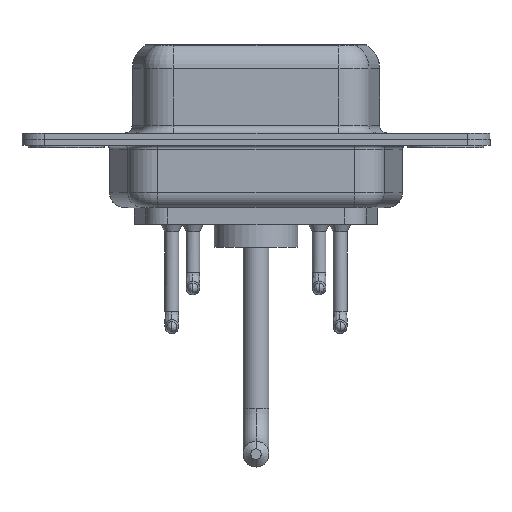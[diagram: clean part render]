
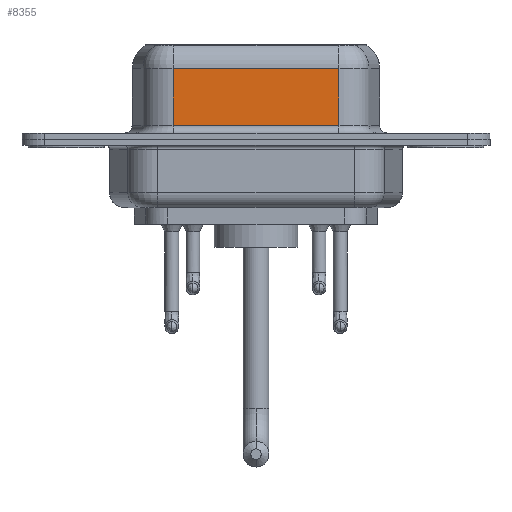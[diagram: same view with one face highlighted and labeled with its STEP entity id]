
A CAD part, front view. The second image highlights one B-rep face of the part: STEP entity #8355.
In plain terms, the highlighted planar face has unit normal (0, -1, 0).
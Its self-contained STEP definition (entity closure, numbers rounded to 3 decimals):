
#8 = CARTESIAN_POINT ( 'NONE',  ( 7.038, -3.95, 6.4 ) ) ;
#379 = CARTESIAN_POINT ( 'NONE',  ( 7.038, -3.95, 4.65 ) ) ;
#430 = CARTESIAN_POINT ( 'NONE',  ( 17.962, -3.95, 6.4 ) ) ;
#712 = DIRECTION ( 'NONE',  ( 0., 1., 0. ) ) ;
#1523 = VECTOR ( 'NONE', #1785, 1000. ) ;
#1714 = CARTESIAN_POINT ( 'NONE',  ( 17.962, -3.95, 0.9 ) ) ;
#1785 = DIRECTION ( 'NONE',  ( 1., 0., 0. ) ) ;
#1871 = VERTEX_POINT ( 'NONE', #10115 ) ;
#1980 = CARTESIAN_POINT ( 'NONE',  ( 17.962, -3.95, 0.9 ) ) ;
#2052 = CARTESIAN_POINT ( 'NONE',  ( 7.038, -3.95, 0.9 ) ) ;
#2303 = VECTOR ( 'NONE', #9220, 1000. ) ;
#2656 = ORIENTED_EDGE ( 'NONE', *, *, #6522, .T. ) ;
#2661 = PLANE ( 'NONE',  #5968 ) ;
#2899 = VERTEX_POINT ( 'NONE', #1980 ) ;
#2935 = FACE_OUTER_BOUND ( 'NONE', #12655, .T. ) ;
#3469 = LINE ( 'NONE', #430, #2303 ) ;
#4029 = DIRECTION ( 'NONE',  ( -1., 0., 0. ) ) ;
#4490 = DIRECTION ( 'NONE',  ( 0., 0., -1. ) ) ;
#4768 = EDGE_CURVE ( 'NONE', #1871, #10885, #14485, .T. ) ;
#4864 = ORIENTED_EDGE ( 'NONE', *, *, #9288, .T. ) ;
#5716 = LINE ( 'NONE', #8, #10631 ) ;
#5968 = AXIS2_PLACEMENT_3D ( 'NONE', #8224, #712, #4029 ) ;
#6522 = EDGE_CURVE ( 'NONE', #10885, #6882, #5716, .T. ) ;
#6639 = CARTESIAN_POINT ( 'NONE',  ( 17.962, -3.95, 4.65 ) ) ;
#6882 = VERTEX_POINT ( 'NONE', #2052 ) ;
#7451 = ORIENTED_EDGE ( 'NONE', *, *, #4768, .T. ) ;
#8224 = CARTESIAN_POINT ( 'NONE',  ( 17.962, -3.95, 6.4 ) ) ;
#8355 = ADVANCED_FACE ( 'NONE', ( #2935 ), #2661, .F. ) ;
#9220 = DIRECTION ( 'NONE',  ( 0., 0., -1. ) ) ;
#9288 = EDGE_CURVE ( 'NONE', #6882, #2899, #12790, .T. ) ;
#10108 = VECTOR ( 'NONE', #13233, 1000. ) ;
#10115 = CARTESIAN_POINT ( 'NONE',  ( 17.962, -3.95, 4.65 ) ) ;
#10631 = VECTOR ( 'NONE', #4490, 1000. ) ;
#10885 = VERTEX_POINT ( 'NONE', #379 ) ;
#10919 = ORIENTED_EDGE ( 'NONE', *, *, #11341, .F. ) ;
#11341 = EDGE_CURVE ( 'NONE', #1871, #2899, #3469, .T. ) ;
#12655 = EDGE_LOOP ( 'NONE', ( #10919, #7451, #2656, #4864 ) ) ;
#12790 = LINE ( 'NONE', #1714, #1523 ) ;
#13233 = DIRECTION ( 'NONE',  ( -1., 0., 0. ) ) ;
#14485 = LINE ( 'NONE', #6639, #10108 ) ;
